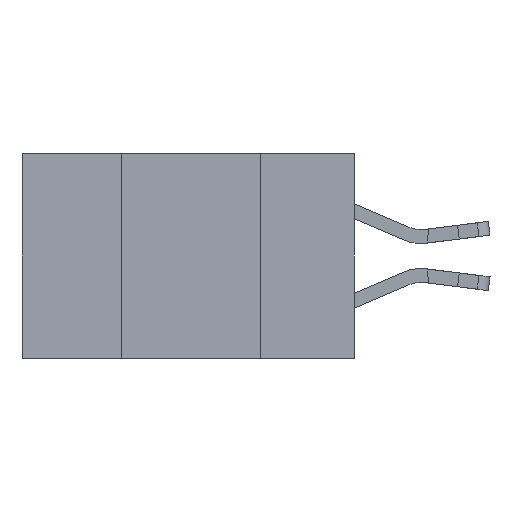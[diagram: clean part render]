
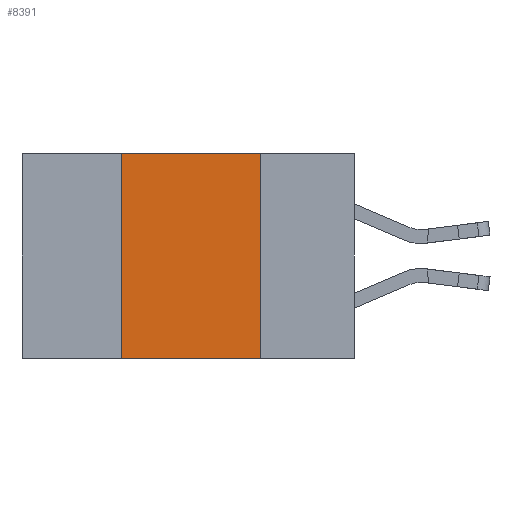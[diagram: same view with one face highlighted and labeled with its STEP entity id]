
A CAD part, left-side view. The second image highlights one B-rep face of the part: STEP entity #8391.
In plain terms, the highlighted planar face has unit normal (-1, 0, 0).
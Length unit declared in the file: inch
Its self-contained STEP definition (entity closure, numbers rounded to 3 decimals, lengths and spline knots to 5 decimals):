
#1002 = VERTEX_POINT ( 'NONE', #10638 ) ;
#1420 = DIRECTION ( 'NONE',  ( 0., -1., 0. ) ) ;
#1434 = CARTESIAN_POINT ( 'NONE',  ( 0., 0.6, -0.37 ) ) ;
#1557 = EDGE_CURVE ( 'NONE', #5747, #1002, #8690, .T. ) ;
#1625 = FACE_OUTER_BOUND ( 'NONE', #5676, .T. ) ;
#1740 = LINE ( 'NONE', #4373, #5044 ) ;
#1942 = VECTOR ( 'NONE', #2024, 39.37008 ) ;
#1966 = VECTOR ( 'NONE', #1420, 39.37008 ) ;
#2024 = DIRECTION ( 'NONE',  ( 0., 0., 1. ) ) ;
#2059 = CARTESIAN_POINT ( 'NONE',  ( 0., 0.42, -0.37 ) ) ;
#2386 = EDGE_CURVE ( 'NONE', #5747, #7712, #5684, .T. ) ;
#2626 = ORIENTED_EDGE ( 'NONE', *, *, #1557, .T. ) ;
#3192 = EDGE_CURVE ( 'NONE', #7712, #15327, #1740, .T. ) ;
#4002 = ORIENTED_EDGE ( 'NONE', *, *, #4054, .F. ) ;
#4054 = EDGE_CURVE ( 'NONE', #15327, #1002, #12044, .T. ) ;
#4209 = DIRECTION ( 'NONE',  ( 0., 0., -1. ) ) ;
#4373 = CARTESIAN_POINT ( 'NONE',  ( 0., 0.6, 0. ) ) ;
#4543 = CARTESIAN_POINT ( 'NONE',  ( 0., 0.17, -0.37 ) ) ;
#4682 = DIRECTION ( 'NONE',  ( 0., -1., 0. ) ) ;
#5044 = VECTOR ( 'NONE', #4682, 39.37008 ) ;
#5405 = CARTESIAN_POINT ( 'NONE',  ( 0., 0.17, 0. ) ) ;
#5594 = ORIENTED_EDGE ( 'NONE', *, *, #3192, .F. ) ;
#5676 = EDGE_LOOP ( 'NONE', ( #4002, #5594, #12999, #2626 ) ) ;
#5684 = LINE ( 'NONE', #2059, #1942 ) ;
#5747 = VERTEX_POINT ( 'NONE', #10180 ) ;
#6692 = VECTOR ( 'NONE', #4209, 39.37008 ) ;
#7712 = VERTEX_POINT ( 'NONE', #14782 ) ;
#8391 = ADVANCED_FACE ( 'NONE', ( #1625 ), #13826, .F. ) ;
#8690 = LINE ( 'NONE', #1434, #1966 ) ;
#10180 = CARTESIAN_POINT ( 'NONE',  ( 0., 0.42, -0.37 ) ) ;
#10638 = CARTESIAN_POINT ( 'NONE',  ( 0., 0.17, -0.37 ) ) ;
#11641 = AXIS2_PLACEMENT_3D ( 'NONE', #13805, #13692, #13679 ) ;
#12044 = LINE ( 'NONE', #4543, #6692 ) ;
#12999 = ORIENTED_EDGE ( 'NONE', *, *, #2386, .F. ) ;
#13679 = DIRECTION ( 'NONE',  ( 0., 0., -1. ) ) ;
#13692 = DIRECTION ( 'NONE',  ( 1., 0., 0. ) ) ;
#13805 = CARTESIAN_POINT ( 'NONE',  ( 0., 0.6, 0. ) ) ;
#13826 = PLANE ( 'NONE',  #11641 ) ;
#14782 = CARTESIAN_POINT ( 'NONE',  ( 0., 0.42, 0. ) ) ;
#15327 = VERTEX_POINT ( 'NONE', #5405 ) ;
